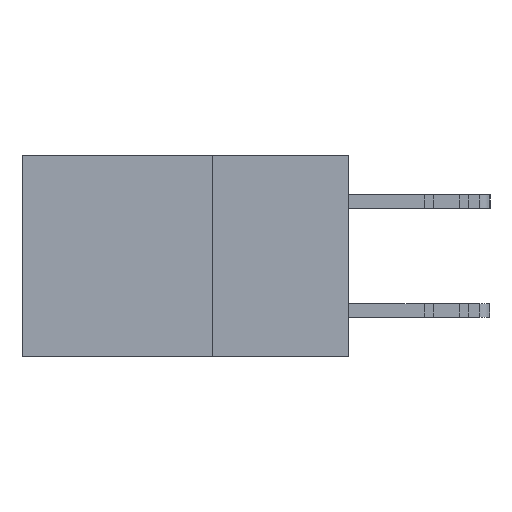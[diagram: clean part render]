
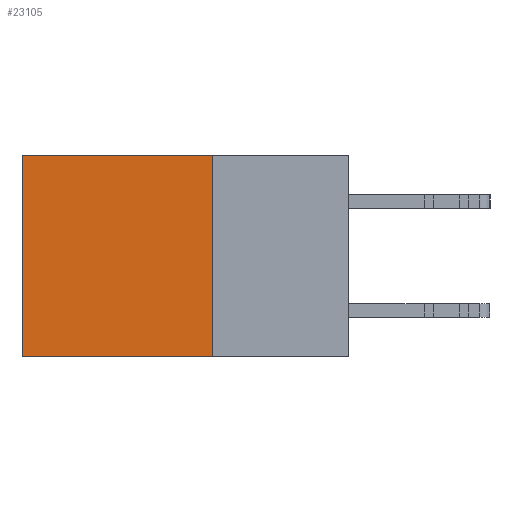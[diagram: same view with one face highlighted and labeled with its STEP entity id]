
A CAD part, left-side view. The second image highlights one B-rep face of the part: STEP entity #23105.
In plain terms, the highlighted planar face has unit normal (-1, 0, 0).
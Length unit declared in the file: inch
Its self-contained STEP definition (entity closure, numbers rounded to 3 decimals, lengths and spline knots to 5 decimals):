
#141 = DIRECTION ( 'NONE',  ( 0., 1., 0. ) ) ;
#424 = CARTESIAN_POINT ( 'NONE',  ( 0.2615, 0.25, -0.37 ) ) ;
#946 = VERTEX_POINT ( 'NONE', #12618 ) ;
#2580 = VERTEX_POINT ( 'NONE', #17755 ) ;
#3129 = VERTEX_POINT ( 'NONE', #20770 ) ;
#4116 = DIRECTION ( 'NONE',  ( 0., 0., -1. ) ) ;
#5715 = EDGE_CURVE ( 'NONE', #3129, #2580, #13651, .T. ) ;
#5723 = CARTESIAN_POINT ( 'NONE',  ( 0.2615, 0.6, 0. ) ) ;
#5855 = EDGE_CURVE ( 'NONE', #3129, #7024, #17435, .T. ) ;
#6366 = DIRECTION ( 'NONE',  ( 1., 0., 0. ) ) ;
#6558 = AXIS2_PLACEMENT_3D ( 'NONE', #424, #6366, #4116 ) ;
#6601 = EDGE_CURVE ( 'NONE', #2580, #946, #14428, .T. ) ;
#6949 = ORIENTED_EDGE ( 'NONE', *, *, #5715, .F. ) ;
#7024 = VERTEX_POINT ( 'NONE', #5723 ) ;
#7973 = CARTESIAN_POINT ( 'NONE',  ( 0.2615, 0.25, -0.37 ) ) ;
#11569 = VECTOR ( 'NONE', #15665, 39.37008 ) ;
#12618 = CARTESIAN_POINT ( 'NONE',  ( 0.2615, 0.6, -0.37 ) ) ;
#13651 = LINE ( 'NONE', #7973, #11569 ) ;
#14428 = LINE ( 'NONE', #20097, #22518 ) ;
#15665 = DIRECTION ( 'NONE',  ( 0., 0., -1. ) ) ;
#15714 = FACE_OUTER_BOUND ( 'NONE', #19998, .T. ) ;
#17435 = LINE ( 'NONE', #21226, #18465 ) ;
#17722 = ORIENTED_EDGE ( 'NONE', *, *, #24421, .T. ) ;
#17755 = CARTESIAN_POINT ( 'NONE',  ( 0.2615, 0.25, -0.37 ) ) ;
#17826 = DIRECTION ( 'NONE',  ( 0., 1., 0. ) ) ;
#18465 = VECTOR ( 'NONE', #141, 39.37008 ) ;
#18986 = VECTOR ( 'NONE', #24070, 39.37008 ) ;
#19998 = EDGE_LOOP ( 'NONE', ( #17722, #20771, #6949, #23338 ) ) ;
#20097 = CARTESIAN_POINT ( 'NONE',  ( 0.2615, 0.25, -0.37 ) ) ;
#20770 = CARTESIAN_POINT ( 'NONE',  ( 0.2615, 0.25, 0. ) ) ;
#20771 = ORIENTED_EDGE ( 'NONE', *, *, #6601, .F. ) ;
#21226 = CARTESIAN_POINT ( 'NONE',  ( 0.2615, 0.25, 0. ) ) ;
#22052 = LINE ( 'NONE', #22302, #18986 ) ;
#22302 = CARTESIAN_POINT ( 'NONE',  ( 0.2615, 0.6, -0.37 ) ) ;
#22518 = VECTOR ( 'NONE', #17826, 39.37008 ) ;
#23105 = ADVANCED_FACE ( 'NONE', ( #15714 ), #23649, .F. ) ;
#23338 = ORIENTED_EDGE ( 'NONE', *, *, #5855, .T. ) ;
#23649 = PLANE ( 'NONE',  #6558 ) ;
#24070 = DIRECTION ( 'NONE',  ( 0., 0., -1. ) ) ;
#24421 = EDGE_CURVE ( 'NONE', #7024, #946, #22052, .T. ) ;
